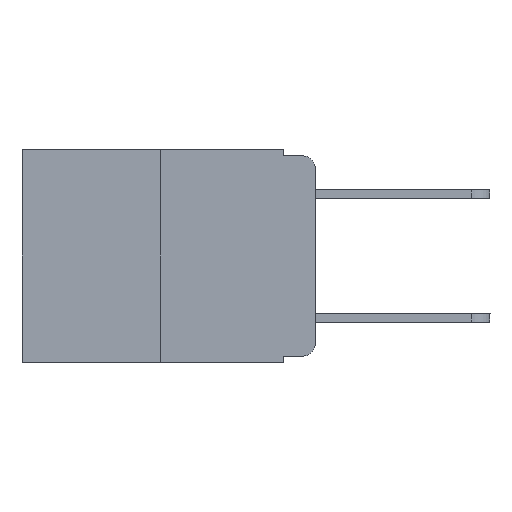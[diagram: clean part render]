
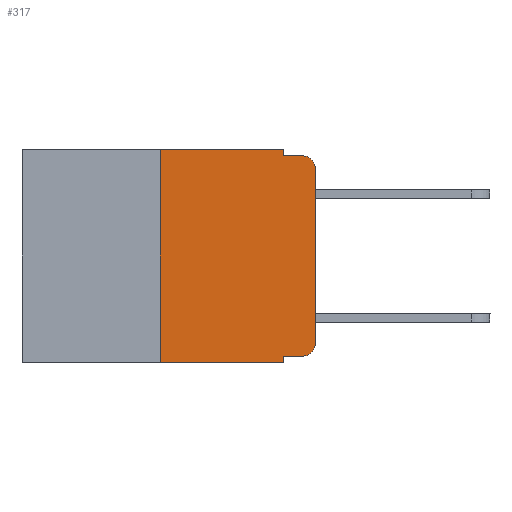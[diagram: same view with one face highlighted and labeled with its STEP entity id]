
A CAD part, left-side view. The second image highlights one B-rep face of the part: STEP entity #317.
In plain terms, the highlighted planar face has unit normal (-1, 0, 0).
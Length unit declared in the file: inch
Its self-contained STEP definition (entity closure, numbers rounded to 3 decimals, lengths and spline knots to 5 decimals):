
#61 = EDGE_CURVE ( 'NONE', #12819, #13301, #6160, .T. ) ;
#212 = CARTESIAN_POINT ( 'NONE',  ( 0., 0.02, -0.313 ) ) ;
#267 = CARTESIAN_POINT ( 'NONE',  ( 0., 0.473, 0. ) ) ;
#275 = CARTESIAN_POINT ( 'NONE',  ( 0., 0.051, 0. ) ) ;
#291 = EDGE_CURVE ( 'NONE', #13381, #11355, #12040, .T. ) ;
#317 = ADVANCED_FACE ( 'NONE', ( #3764 ), #1012, .F. ) ;
#431 = EDGE_CURVE ( 'NONE', #6779, #12819, #2255, .T. ) ;
#519 = CARTESIAN_POINT ( 'NONE',  ( 0., 0.02, -0.03 ) ) ;
#723 = VECTOR ( 'NONE', #8819, 39.37008 ) ;
#1005 = CARTESIAN_POINT ( 'NONE',  ( 0., 0.25, -0.343 ) ) ;
#1012 = PLANE ( 'NONE',  #4685 ) ;
#1042 = DIRECTION ( 'NONE',  ( 0., -1., 0. ) ) ;
#1542 = LINE ( 'NONE', #8683, #723 ) ;
#2040 = ORIENTED_EDGE ( 'NONE', *, *, #3368, .T. ) ;
#2184 = DIRECTION ( 'NONE',  ( 0., 0., -1. ) ) ;
#2252 = VECTOR ( 'NONE', #7462, 39.37008 ) ;
#2255 = LINE ( 'NONE', #3659, #10529 ) ;
#2294 = CARTESIAN_POINT ( 'NONE',  ( 0., 0.02, -0.01 ) ) ;
#2543 = VERTEX_POINT ( 'NONE', #1005 ) ;
#2732 = DIRECTION ( 'NONE',  ( -1., 0., 0. ) ) ;
#2827 = CARTESIAN_POINT ( 'NONE',  ( 0., 0.051, -0.343 ) ) ;
#2930 = LINE ( 'NONE', #12810, #13594 ) ;
#3033 = ORIENTED_EDGE ( 'NONE', *, *, #431, .F. ) ;
#3247 = ORIENTED_EDGE ( 'NONE', *, *, #4495, .F. ) ;
#3267 = CARTESIAN_POINT ( 'NONE',  ( 0., 0., 0. ) ) ;
#3368 = EDGE_CURVE ( 'NONE', #13298, #8687, #13956, .T. ) ;
#3395 = CARTESIAN_POINT ( 'NONE',  ( 0., 0.02, -0.333 ) ) ;
#3416 = ORIENTED_EDGE ( 'NONE', *, *, #61, .F. ) ;
#3582 = ORIENTED_EDGE ( 'NONE', *, *, #291, .T. ) ;
#3659 = CARTESIAN_POINT ( 'NONE',  ( 0., 0.473, 0. ) ) ;
#3764 = FACE_OUTER_BOUND ( 'NONE', #4556, .T. ) ;
#4025 = ORIENTED_EDGE ( 'NONE', *, *, #4212, .F. ) ;
#4212 = EDGE_CURVE ( 'NONE', #13381, #4693, #2930, .T. ) ;
#4270 = EDGE_CURVE ( 'NONE', #5113, #13298, #4282, .T. ) ;
#4282 = LINE ( 'NONE', #3267, #2252 ) ;
#4364 = CARTESIAN_POINT ( 'NONE',  ( 0., 0.051, -0.01 ) ) ;
#4495 = EDGE_CURVE ( 'NONE', #13301, #8687, #5291, .T. ) ;
#4556 = EDGE_LOOP ( 'NONE', ( #8286, #2040, #3247, #3416, #3033, #6432, #8505, #4025, #3582, #9482 ) ) ;
#4685 = AXIS2_PLACEMENT_3D ( 'NONE', #267, #9697, #10782 ) ;
#4693 = VERTEX_POINT ( 'NONE', #2827 ) ;
#5113 = VERTEX_POINT ( 'NONE', #13112 ) ;
#5291 = LINE ( 'NONE', #8755, #7517 ) ;
#5531 = EDGE_CURVE ( 'NONE', #11355, #5113, #6802, .T. ) ;
#5665 = EDGE_CURVE ( 'NONE', #2543, #4693, #1542, .T. ) ;
#5798 = DIRECTION ( 'NONE',  ( 0., 0., 1. ) ) ;
#6160 = LINE ( 'NONE', #7953, #7020 ) ;
#6432 = ORIENTED_EDGE ( 'NONE', *, *, #8393, .F. ) ;
#6779 = VERTEX_POINT ( 'NONE', #9390 ) ;
#6795 = CARTESIAN_POINT ( 'NONE',  ( 0., 0.051, -0.333 ) ) ;
#6802 = CIRCLE ( 'NONE', #10436, 0.02 ) ;
#6848 = LINE ( 'NONE', #12388, #9360 ) ;
#7020 = VECTOR ( 'NONE', #11249, 39.37008 ) ;
#7364 = CARTESIAN_POINT ( 'NONE',  ( 0., 0., -0.03 ) ) ;
#7462 = DIRECTION ( 'NONE',  ( 0., 0., 1. ) ) ;
#7517 = VECTOR ( 'NONE', #8398, 39.37008 ) ;
#7608 = DIRECTION ( 'NONE',  ( -1., 0., 0. ) ) ;
#7799 = DIRECTION ( 'NONE',  ( 0., 0., -1. ) ) ;
#7953 = CARTESIAN_POINT ( 'NONE',  ( 0., 0.051, 0. ) ) ;
#8286 = ORIENTED_EDGE ( 'NONE', *, *, #4270, .T. ) ;
#8393 = EDGE_CURVE ( 'NONE', #2543, #6779, #6848, .T. ) ;
#8398 = DIRECTION ( 'NONE',  ( 0., -1., 0. ) ) ;
#8505 = ORIENTED_EDGE ( 'NONE', *, *, #5665, .T. ) ;
#8524 = VECTOR ( 'NONE', #1042, 39.37008 ) ;
#8683 = CARTESIAN_POINT ( 'NONE',  ( 0., 0.473, -0.343 ) ) ;
#8687 = VERTEX_POINT ( 'NONE', #2294 ) ;
#8755 = CARTESIAN_POINT ( 'NONE',  ( 0., 0.051, -0.01 ) ) ;
#8819 = DIRECTION ( 'NONE',  ( 0., -1., 0. ) ) ;
#9360 = VECTOR ( 'NONE', #5798, 39.37008 ) ;
#9390 = CARTESIAN_POINT ( 'NONE',  ( 0., 0.25, 0. ) ) ;
#9482 = ORIENTED_EDGE ( 'NONE', *, *, #5531, .T. ) ;
#9697 = DIRECTION ( 'NONE',  ( 1., 0., 0. ) ) ;
#10436 = AXIS2_PLACEMENT_3D ( 'NONE', #212, #7608, #7799 ) ;
#10529 = VECTOR ( 'NONE', #12288, 39.37008 ) ;
#10782 = DIRECTION ( 'NONE',  ( 0., 0., -1. ) ) ;
#11249 = DIRECTION ( 'NONE',  ( 0., 0., -1. ) ) ;
#11355 = VERTEX_POINT ( 'NONE', #3395 ) ;
#11357 = DIRECTION ( 'NONE',  ( 0., 0., -1. ) ) ;
#11584 = AXIS2_PLACEMENT_3D ( 'NONE', #519, #2732, #11357 ) ;
#11789 = CARTESIAN_POINT ( 'NONE',  ( 0., 0.051, -0.333 ) ) ;
#12040 = LINE ( 'NONE', #11789, #8524 ) ;
#12288 = DIRECTION ( 'NONE',  ( 0., -1., 0. ) ) ;
#12388 = CARTESIAN_POINT ( 'NONE',  ( 0., 0.25, 0. ) ) ;
#12810 = CARTESIAN_POINT ( 'NONE',  ( 0., 0.051, 0. ) ) ;
#12819 = VERTEX_POINT ( 'NONE', #275 ) ;
#13112 = CARTESIAN_POINT ( 'NONE',  ( 0., 0., -0.313 ) ) ;
#13298 = VERTEX_POINT ( 'NONE', #7364 ) ;
#13301 = VERTEX_POINT ( 'NONE', #4364 ) ;
#13381 = VERTEX_POINT ( 'NONE', #6795 ) ;
#13594 = VECTOR ( 'NONE', #2184, 39.37008 ) ;
#13956 = CIRCLE ( 'NONE', #11584, 0.02 ) ;
